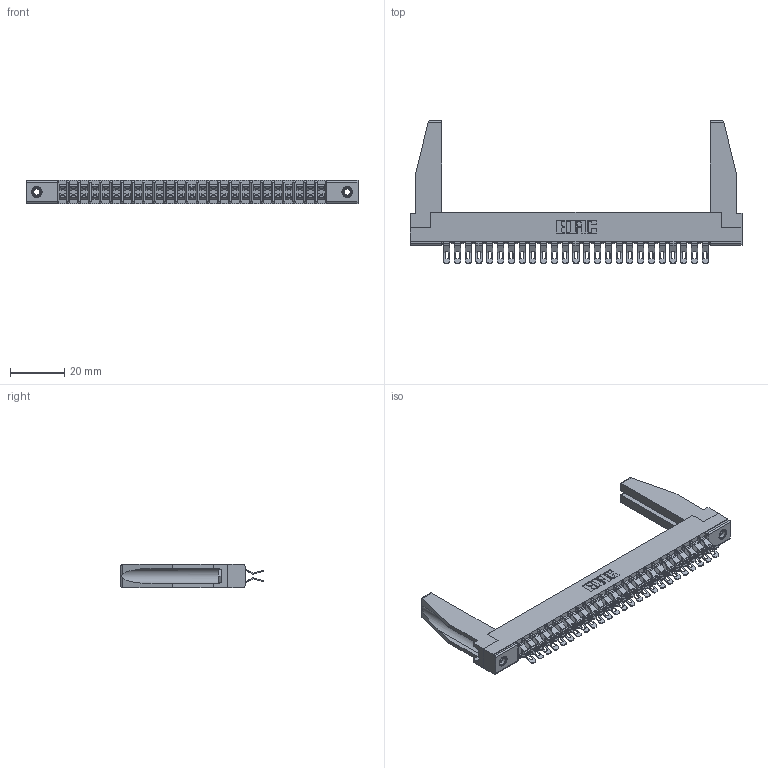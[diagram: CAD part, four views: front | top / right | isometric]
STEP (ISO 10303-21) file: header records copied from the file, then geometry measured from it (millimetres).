
FILE_DESCRIPTION (( 'STEP AP203' ), '1' );
FILE_NAME ('307-050-555-278.STEP', '2019-09-06T11:17:30', ( '' ), ( '' ), 'SwSTEP 2.0', 'SolidWorks 2016', '' );
FILE_SCHEMA (( 'CONFIG_CONTROL_DESIGN' ));
Length unit declared in the file: inch
Products named in the file (5): 307 Part_.156 Dia Mounting Holes; 307-220-078; 307-050-555-278; 307-290-001_555; 345-250-001_345-250-001-102
Assembly tree (55 placements, depth 2):
  307-050-555-278
    307 Part_.156 Dia Mounting Holes
    307-290-001_555  x50
    307-220-078  x2
    345-250-001_345-250-001-102  x2
Bounding box: 122.07 x 52.45 x 8.71 mm (x, y, z)
Volume: 12126.8 mm3; surface area: 19169 mm2
Topology: 55 solids, 55 shells, 3324 faces, 9703 edges, 6322 vertices
Faces by surface type: plane 1854, cylinder 1402, sphere 52, cone 12, torus 4
Entity records: 27304 total; most frequent: CARTESIAN_POINT 4487, ORIENTED_EDGE 4406, DIRECTION 4363, EDGE_CURVE 2203, LINE 1675, VECTOR 1675, VERTEX_POINT 1426, AXIS2_PLACEMENT_3D 1344
